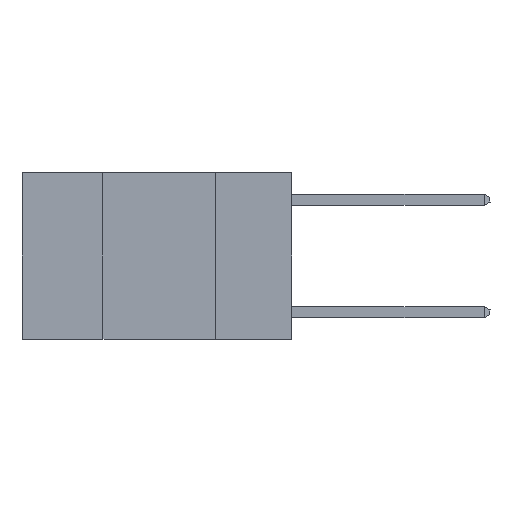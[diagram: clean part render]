
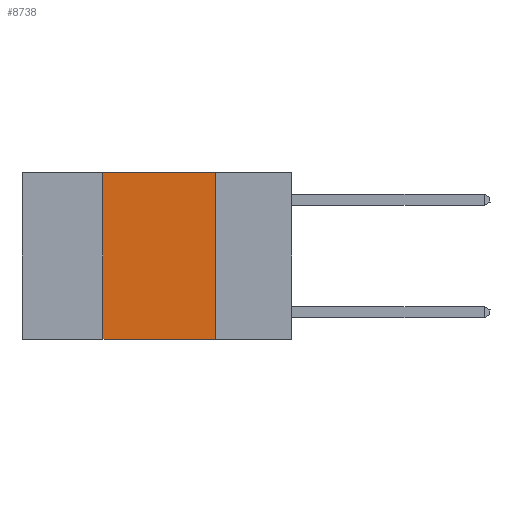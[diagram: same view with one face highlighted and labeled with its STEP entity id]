
A CAD part, left-side view. The second image highlights one B-rep face of the part: STEP entity #8738.
In plain terms, the highlighted planar face has unit normal (-1, 0, 0).
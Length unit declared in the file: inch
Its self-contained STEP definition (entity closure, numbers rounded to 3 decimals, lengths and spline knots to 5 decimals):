
#741 = CARTESIAN_POINT ( 'NONE',  ( 0., 0.42, 0. ) ) ;
#826 = EDGE_CURVE ( 'NONE', #16455, #9726, #22557, .T. ) ;
#1174 = ORIENTED_EDGE ( 'NONE', *, *, #5317, .F. ) ;
#2472 = CARTESIAN_POINT ( 'NONE',  ( 0., 0.42, -0.37 ) ) ;
#5317 = EDGE_CURVE ( 'NONE', #15245, #11165, #7125, .T. ) ;
#7125 = LINE ( 'NONE', #9561, #21248 ) ;
#7380 = CARTESIAN_POINT ( 'NONE',  ( 0., 0.6, -0.37 ) ) ;
#8725 = CARTESIAN_POINT ( 'NONE',  ( 0., 0.6, 0. ) ) ;
#8738 = ADVANCED_FACE ( 'NONE', ( #8996 ), #19473, .F. ) ;
#8822 = AXIS2_PLACEMENT_3D ( 'NONE', #8725, #17344, #26113 ) ;
#8996 = FACE_OUTER_BOUND ( 'NONE', #9902, .T. ) ;
#9270 = DIRECTION ( 'NONE',  ( 0., -1., 0. ) ) ;
#9561 = CARTESIAN_POINT ( 'NONE',  ( 0., 0.6, 0. ) ) ;
#9726 = VERTEX_POINT ( 'NONE', #16083 ) ;
#9902 = EDGE_LOOP ( 'NONE', ( #11423, #1174, #14306, #23398 ) ) ;
#11165 = VERTEX_POINT ( 'NONE', #14218 ) ;
#11423 = ORIENTED_EDGE ( 'NONE', *, *, #21705, .F. ) ;
#11657 = DIRECTION ( 'NONE',  ( 0., -1., 0. ) ) ;
#11985 = VECTOR ( 'NONE', #21493, 39.37008 ) ;
#12036 = CARTESIAN_POINT ( 'NONE',  ( 0., 0.17, 0. ) ) ;
#13862 = DIRECTION ( 'NONE',  ( 0., 0., -1. ) ) ;
#14218 = CARTESIAN_POINT ( 'NONE',  ( 0., 0.17, 0. ) ) ;
#14306 = ORIENTED_EDGE ( 'NONE', *, *, #24626, .F. ) ;
#14567 = LINE ( 'NONE', #23469, #11985 ) ;
#15245 = VERTEX_POINT ( 'NONE', #741 ) ;
#16083 = CARTESIAN_POINT ( 'NONE',  ( 0., 0.17, -0.37 ) ) ;
#16455 = VERTEX_POINT ( 'NONE', #2472 ) ;
#17344 = DIRECTION ( 'NONE',  ( 1., 0., 0. ) ) ;
#18537 = VECTOR ( 'NONE', #13862, 39.37008 ) ;
#19473 = PLANE ( 'NONE',  #8822 ) ;
#20127 = VECTOR ( 'NONE', #11657, 39.37008 ) ;
#21248 = VECTOR ( 'NONE', #9270, 39.37008 ) ;
#21493 = DIRECTION ( 'NONE',  ( 0., 0., 1. ) ) ;
#21705 = EDGE_CURVE ( 'NONE', #11165, #9726, #25053, .T. ) ;
#22557 = LINE ( 'NONE', #7380, #20127 ) ;
#23398 = ORIENTED_EDGE ( 'NONE', *, *, #826, .T. ) ;
#23469 = CARTESIAN_POINT ( 'NONE',  ( 0., 0.42, 0. ) ) ;
#24626 = EDGE_CURVE ( 'NONE', #16455, #15245, #14567, .T. ) ;
#25053 = LINE ( 'NONE', #12036, #18537 ) ;
#26113 = DIRECTION ( 'NONE',  ( 0., 0., -1. ) ) ;
